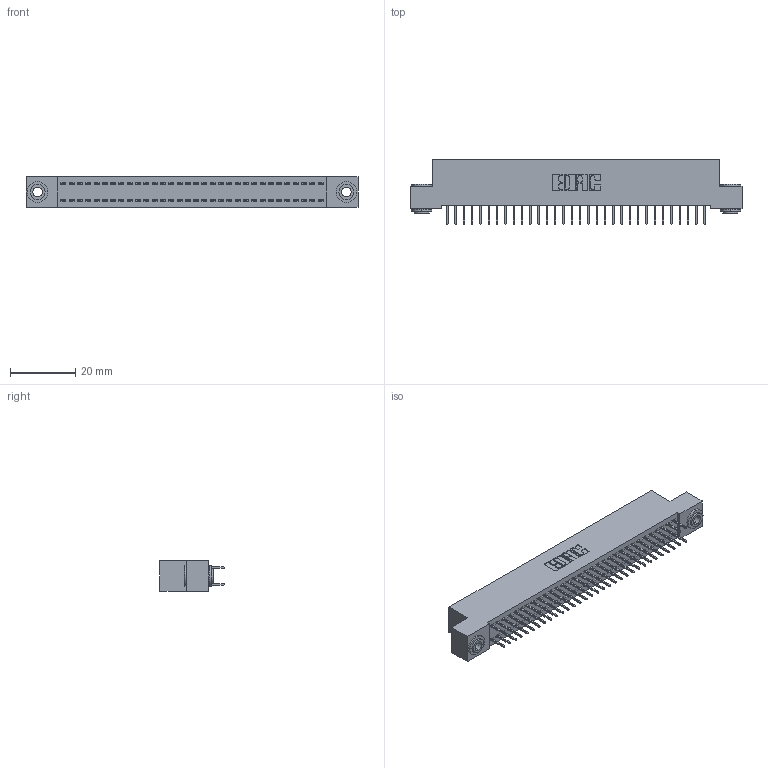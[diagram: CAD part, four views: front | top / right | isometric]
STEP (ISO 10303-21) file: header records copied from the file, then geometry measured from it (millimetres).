
FILE_DESCRIPTION (( 'STEP AP203' ), '1' );
FILE_NAME ('392-064-524-203.STEP', '2019-10-09T10:44:50', ( '' ), ( '' ), 'SwSTEP 2.0', 'SolidWorks 2016', '' );
FILE_SCHEMA (( 'CONFIG_CONTROL_DESIGN' ));
Length unit declared in the file: inch
Products named in the file (4): 392-064-524-203; 342 Part_.156 TH; 345-292-001_345-293-124; 342-250-002_345-250-002-102
Assembly tree (67 placements, depth 2):
  392-064-524-203
    342 Part_.156 TH
    345-292-001_345-293-124  x64
    342-250-002_345-250-002-102  x2
Bounding box: 101.6 x 19.69 x 9.4 mm (x, y, z)
Volume: 9007.4 mm3; surface area: 14377.5 mm2
Topology: 67 solids, 67 shells, 3732 faces, 10551 edges, 6774 vertices
Faces by surface type: plane 2764, cylinder 960, cone 8
Entity records: 22472 total; most frequent: CARTESIAN_POINT 3709, ORIENTED_EDGE 3638, DIRECTION 3221, EDGE_CURVE 1819, VECTOR 1671, LINE 1671, VERTEX_POINT 1206, AXIS2_PLACEMENT_3D 775
